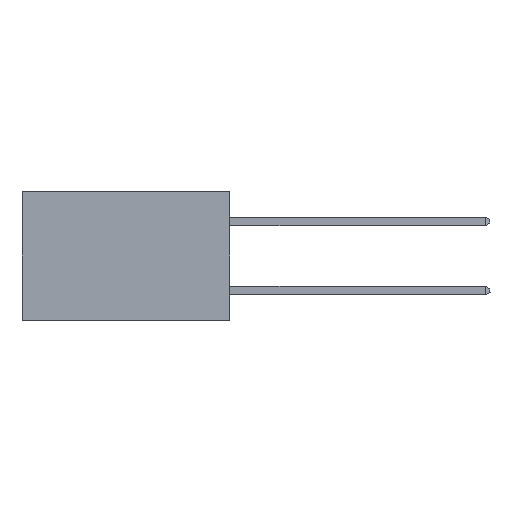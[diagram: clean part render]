
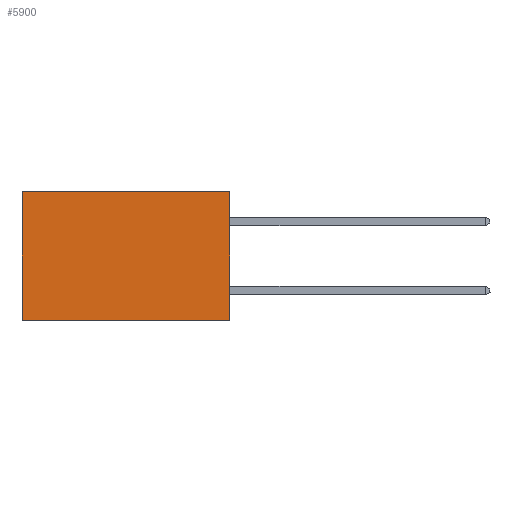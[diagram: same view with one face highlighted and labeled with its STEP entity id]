
A CAD part, left-side view. The second image highlights one B-rep face of the part: STEP entity #5900.
In plain terms, the highlighted planar face has unit normal (-1, 0, 0).
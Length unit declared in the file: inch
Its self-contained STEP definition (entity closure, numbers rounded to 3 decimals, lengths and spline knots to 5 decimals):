
#137 = VERTEX_POINT ( 'NONE', #11021 ) ;
#2164 = DIRECTION ( 'NONE',  ( 0., 0., -1. ) ) ;
#2866 = EDGE_CURVE ( 'NONE', #3593, #137, #8335, .T. ) ;
#3593 = VERTEX_POINT ( 'NONE', #10132 ) ;
#3767 = DIRECTION ( 'NONE',  ( 0., 0., -1. ) ) ;
#3776 = EDGE_CURVE ( 'NONE', #17162, #15484, #12311, .T. ) ;
#5900 = ADVANCED_FACE ( 'NONE', ( #18499 ), #17558, .F. ) ;
#6707 = LINE ( 'NONE', #17673, #17004 ) ;
#7562 = CARTESIAN_POINT ( 'NONE',  ( 0.298, 0., 0. ) ) ;
#7606 = ORIENTED_EDGE ( 'NONE', *, *, #2866, .T. ) ;
#7957 = CARTESIAN_POINT ( 'NONE',  ( 0.298, 0., -0.37 ) ) ;
#8335 = LINE ( 'NONE', #12184, #8757 ) ;
#8757 = VECTOR ( 'NONE', #15037, 39.37008 ) ;
#8890 = CARTESIAN_POINT ( 'NONE',  ( 0.298, 0., -0.37 ) ) ;
#9005 = DIRECTION ( 'NONE',  ( 1., 0., 0. ) ) ;
#9293 = EDGE_LOOP ( 'NONE', ( #12828, #13602, #10654, #7606 ) ) ;
#9646 = VECTOR ( 'NONE', #15049, 39.37008 ) ;
#9766 = VECTOR ( 'NONE', #3767, 39.37008 ) ;
#10132 = CARTESIAN_POINT ( 'NONE',  ( 0.298, 0., 0. ) ) ;
#10465 = EDGE_CURVE ( 'NONE', #137, #15484, #6707, .T. ) ;
#10654 = ORIENTED_EDGE ( 'NONE', *, *, #12445, .F. ) ;
#11021 = CARTESIAN_POINT ( 'NONE',  ( 0.298, 0.6, 0. ) ) ;
#11674 = CARTESIAN_POINT ( 'NONE',  ( 0.298, 0.6, -0.37 ) ) ;
#12184 = CARTESIAN_POINT ( 'NONE',  ( 0.298, 0., 0. ) ) ;
#12213 = LINE ( 'NONE', #16416, #9766 ) ;
#12311 = LINE ( 'NONE', #7957, #9646 ) ;
#12445 = EDGE_CURVE ( 'NONE', #3593, #17162, #12213, .T. ) ;
#12828 = ORIENTED_EDGE ( 'NONE', *, *, #10465, .T. ) ;
#13602 = ORIENTED_EDGE ( 'NONE', *, *, #3776, .F. ) ;
#15037 = DIRECTION ( 'NONE',  ( 0., 1., 0. ) ) ;
#15049 = DIRECTION ( 'NONE',  ( 0., 1., 0. ) ) ;
#15484 = VERTEX_POINT ( 'NONE', #11674 ) ;
#16416 = CARTESIAN_POINT ( 'NONE',  ( 0.298, 0., 0. ) ) ;
#17004 = VECTOR ( 'NONE', #2164, 39.37008 ) ;
#17162 = VERTEX_POINT ( 'NONE', #8890 ) ;
#17376 = DIRECTION ( 'NONE',  ( 0., 0., -1. ) ) ;
#17556 = AXIS2_PLACEMENT_3D ( 'NONE', #7562, #9005, #17376 ) ;
#17558 = PLANE ( 'NONE',  #17556 ) ;
#17673 = CARTESIAN_POINT ( 'NONE',  ( 0.298, 0.6, 0. ) ) ;
#18499 = FACE_OUTER_BOUND ( 'NONE', #9293, .T. ) ;
